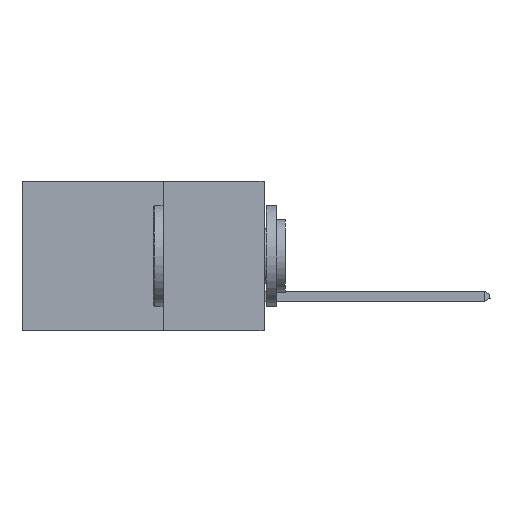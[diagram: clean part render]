
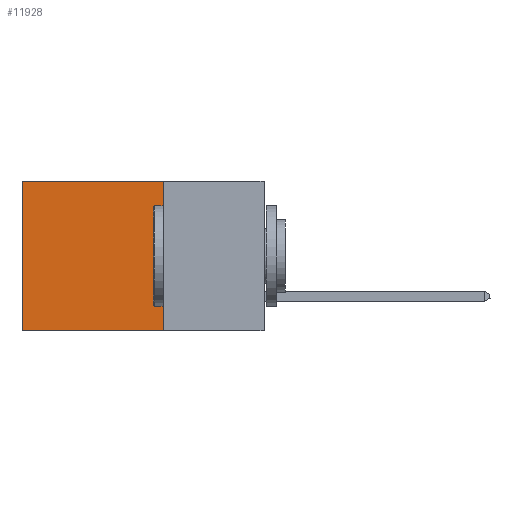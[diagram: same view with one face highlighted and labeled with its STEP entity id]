
A CAD part, left-side view. The second image highlights one B-rep face of the part: STEP entity #11928.
In plain terms, the highlighted planar face has unit normal (-1, 0, 0).
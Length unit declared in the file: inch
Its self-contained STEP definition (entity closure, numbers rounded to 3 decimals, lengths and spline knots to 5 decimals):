
#484 = EDGE_CURVE ( 'NONE', #5971, #4516, #5775, .T. ) ;
#619 = DIRECTION ( 'NONE',  ( 0., 0., -1. ) ) ;
#985 = ORIENTED_EDGE ( 'NONE', *, *, #10873, .T. ) ;
#1038 = LINE ( 'NONE', #13047, #8027 ) ;
#1299 = ORIENTED_EDGE ( 'NONE', *, *, #484, .F. ) ;
#1450 = EDGE_CURVE ( 'NONE', #4461, #4516, #1038, .T. ) ;
#2661 = DIRECTION ( 'NONE',  ( 0., 1., 0. ) ) ;
#2731 = VECTOR ( 'NONE', #2661, 39.37008 ) ;
#2846 = EDGE_CURVE ( 'NONE', #3260, #5971, #13157, .T. ) ;
#3260 = VERTEX_POINT ( 'NONE', #8768 ) ;
#3387 = CARTESIAN_POINT ( 'NONE',  ( 0.2615, 0.25, 0. ) ) ;
#3404 = CARTESIAN_POINT ( 'NONE',  ( 0.2615, 0.25, -0.37 ) ) ;
#4360 = CARTESIAN_POINT ( 'NONE',  ( 0.2615, 0.25, -0.37 ) ) ;
#4461 = VERTEX_POINT ( 'NONE', #11158 ) ;
#4516 = VERTEX_POINT ( 'NONE', #4804 ) ;
#4804 = CARTESIAN_POINT ( 'NONE',  ( 0.2615, 0.6, -0.37 ) ) ;
#5273 = VECTOR ( 'NONE', #7403, 39.37008 ) ;
#5775 = LINE ( 'NONE', #3404, #2731 ) ;
#5857 = CARTESIAN_POINT ( 'NONE',  ( 0.2615, 0.25, -0.37 ) ) ;
#5971 = VERTEX_POINT ( 'NONE', #4360 ) ;
#7403 = DIRECTION ( 'NONE',  ( 0., 0., -1. ) ) ;
#7568 = AXIS2_PLACEMENT_3D ( 'NONE', #5857, #8216, #12803 ) ;
#8027 = VECTOR ( 'NONE', #619, 39.37008 ) ;
#8216 = DIRECTION ( 'NONE',  ( 1., 0., 0. ) ) ;
#8733 = ORIENTED_EDGE ( 'NONE', *, *, #1450, .T. ) ;
#8768 = CARTESIAN_POINT ( 'NONE',  ( 0.2615, 0.25, 0. ) ) ;
#10152 = DIRECTION ( 'NONE',  ( 0., 1., 0. ) ) ;
#10873 = EDGE_CURVE ( 'NONE', #3260, #4461, #13132, .T. ) ;
#11158 = CARTESIAN_POINT ( 'NONE',  ( 0.2615, 0.6, 0. ) ) ;
#11884 = FACE_OUTER_BOUND ( 'NONE', #13588, .T. ) ;
#11928 = ADVANCED_FACE ( 'NONE', ( #11884 ), #13378, .F. ) ;
#12803 = DIRECTION ( 'NONE',  ( 0., 0., -1. ) ) ;
#12956 = CARTESIAN_POINT ( 'NONE',  ( 0.2615, 0.25, -0.37 ) ) ;
#13047 = CARTESIAN_POINT ( 'NONE',  ( 0.2615, 0.6, -0.37 ) ) ;
#13132 = LINE ( 'NONE', #3387, #13868 ) ;
#13157 = LINE ( 'NONE', #12956, #5273 ) ;
#13378 = PLANE ( 'NONE',  #7568 ) ;
#13588 = EDGE_LOOP ( 'NONE', ( #8733, #1299, #14179, #985 ) ) ;
#13868 = VECTOR ( 'NONE', #10152, 39.37008 ) ;
#14179 = ORIENTED_EDGE ( 'NONE', *, *, #2846, .F. ) ;
